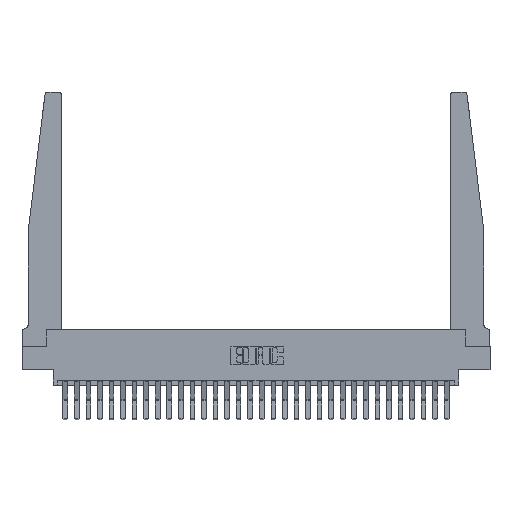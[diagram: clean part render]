
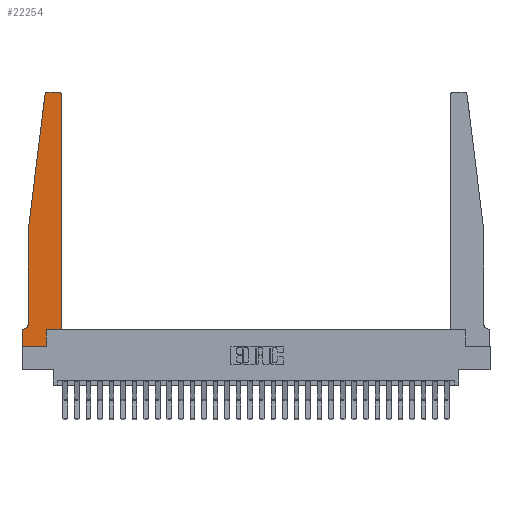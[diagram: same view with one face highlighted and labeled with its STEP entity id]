
A CAD part, top view. The second image highlights one B-rep face of the part: STEP entity #22254.
In plain terms, the highlighted planar face has unit normal (0, 0, 1).
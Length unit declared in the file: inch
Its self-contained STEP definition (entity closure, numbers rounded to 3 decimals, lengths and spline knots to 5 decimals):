
#412 = DIRECTION ( 'NONE',  ( -1., 0., 0. ) ) ;
#1048 = CARTESIAN_POINT ( 'NONE',  ( 0.24675, 2.72367, 0.37 ) ) ;
#1171 = VECTOR ( 'NONE', #17797, 39.37008 ) ;
#1182 = ORIENTED_EDGE ( 'NONE', *, *, #18888, .T. ) ;
#1432 = CARTESIAN_POINT ( 'NONE',  ( 0.015, 0.1875, 0.37 ) ) ;
#1631 = ORIENTED_EDGE ( 'NONE', *, *, #15949, .T. ) ;
#1781 = AXIS2_PLACEMENT_3D ( 'NONE', #4425, #19677, #6575 ) ;
#2222 = PLANE ( 'NONE',  #1781 ) ;
#2535 = EDGE_CURVE ( 'NONE', #12598, #18628, #19215, .T. ) ;
#2574 = CARTESIAN_POINT ( 'NONE',  ( 0.425, 0.18, 0.37 ) ) ;
#3035 = DIRECTION ( 'NONE',  ( 0., 1., 0. ) ) ;
#3255 = VECTOR ( 'NONE', #15378, 39.37008 ) ;
#3931 = LINE ( 'NONE', #6574, #3255 ) ;
#4401 = VERTEX_POINT ( 'NONE', #5819 ) ;
#4425 = CARTESIAN_POINT ( 'NONE',  ( 0., 0.1875, 0.37 ) ) ;
#4804 = ORIENTED_EDGE ( 'NONE', *, *, #23643, .T. ) ;
#4935 = DIRECTION ( 'NONE',  ( 0., -1., 0. ) ) ;
#5178 = VECTOR ( 'NONE', #412, 39.37008 ) ;
#5334 = EDGE_CURVE ( 'NONE', #24561, #4401, #14353, .T. ) ;
#5622 = VERTEX_POINT ( 'NONE', #8802 ) ;
#5819 = CARTESIAN_POINT ( 'NONE',  ( 0.2605, 0.18, 0.37 ) ) ;
#6364 = EDGE_CURVE ( 'NONE', #5622, #7154, #12921, .T. ) ;
#6537 = FACE_OUTER_BOUND ( 'NONE', #28158, .T. ) ;
#6574 = CARTESIAN_POINT ( 'NONE',  ( 0.425, 0.18, 0.37 ) ) ;
#6575 = DIRECTION ( 'NONE',  ( 1., 0., 0. ) ) ;
#7086 = VECTOR ( 'NONE', #15742, 39.37008 ) ;
#7107 = CARTESIAN_POINT ( 'NONE',  ( 0.065, 1.25, 0.37 ) ) ;
#7154 = VERTEX_POINT ( 'NONE', #14189 ) ;
#7252 = CARTESIAN_POINT ( 'NONE',  ( 0.27653, 2.72, 0.37 ) ) ;
#7604 = VECTOR ( 'NONE', #4935, 39.37008 ) ;
#7859 = VECTOR ( 'NONE', #20380, 39.37008 ) ;
#7932 = DIRECTION ( 'NONE',  ( 0., 0., 1. ) ) ;
#8140 = ORIENTED_EDGE ( 'NONE', *, *, #16563, .T. ) ;
#8578 = VERTEX_POINT ( 'NONE', #1432 ) ;
#8802 = CARTESIAN_POINT ( 'NONE',  ( 0.425, 0.18, 0.37 ) ) ;
#9468 = DIRECTION ( 'NONE',  ( 1., 0., 0. ) ) ;
#9746 = CARTESIAN_POINT ( 'NONE',  ( 0.27653, 2.75, 0.37 ) ) ;
#9962 = LINE ( 'NONE', #21421, #20895 ) ;
#11120 = VECTOR ( 'NONE', #24467, 39.37008 ) ;
#11177 = CARTESIAN_POINT ( 'NONE',  ( 0.2605, 0., 0.37 ) ) ;
#11211 = EDGE_CURVE ( 'NONE', #4401, #5622, #3931, .T. ) ;
#11374 = EDGE_CURVE ( 'NONE', #24671, #11467, #23013, .T. ) ;
#11386 = ORIENTED_EDGE ( 'NONE', *, *, #11374, .T. ) ;
#11467 = VERTEX_POINT ( 'NONE', #1048 ) ;
#11608 = CIRCLE ( 'NONE', #27369, 0.05 ) ;
#11744 = VERTEX_POINT ( 'NONE', #21482 ) ;
#11816 = LINE ( 'NONE', #7107, #11120 ) ;
#11883 = CARTESIAN_POINT ( 'NONE',  ( 0.015, 0.2375, 0.37 ) ) ;
#11953 = ORIENTED_EDGE ( 'NONE', *, *, #2535, .T. ) ;
#12598 = VERTEX_POINT ( 'NONE', #24790 ) ;
#12805 = LINE ( 'NONE', #15581, #1171 ) ;
#12921 = LINE ( 'NONE', #2574, #7086 ) ;
#12975 = ORIENTED_EDGE ( 'NONE', *, *, #5334, .T. ) ;
#14073 = DIRECTION ( 'NONE',  ( -1., 0., 0. ) ) ;
#14189 = CARTESIAN_POINT ( 'NONE',  ( 0.425, 2.72, 0.37 ) ) ;
#14353 = LINE ( 'NONE', #16079, #25237 ) ;
#14684 = CARTESIAN_POINT ( 'NONE',  ( 0.395, 2.72, 0.37 ) ) ;
#15039 = LINE ( 'NONE', #15979, #7859 ) ;
#15083 = EDGE_CURVE ( 'NONE', #7154, #11744, #25820, .T. ) ;
#15378 = DIRECTION ( 'NONE',  ( 1., 0., 0. ) ) ;
#15409 = VERTEX_POINT ( 'NONE', #19743 ) ;
#15581 = CARTESIAN_POINT ( 'NONE',  ( 0.065, 0.1875, 0.37 ) ) ;
#15742 = DIRECTION ( 'NONE',  ( 0., 1., 0. ) ) ;
#15809 = CARTESIAN_POINT ( 'NONE',  ( 0.065, 1.25, 0.37 ) ) ;
#15949 = EDGE_CURVE ( 'NONE', #11467, #12598, #11816, .T. ) ;
#15979 = CARTESIAN_POINT ( 'NONE',  ( 0., 0., 0.37 ) ) ;
#16072 = AXIS2_PLACEMENT_3D ( 'NONE', #7252, #22529, #9468 ) ;
#16079 = CARTESIAN_POINT ( 'NONE',  ( 0.2605, 0.18, 0.37 ) ) ;
#16176 = ORIENTED_EDGE ( 'NONE', *, *, #11211, .T. ) ;
#16342 = ORIENTED_EDGE ( 'NONE', *, *, #15083, .T. ) ;
#16563 = EDGE_CURVE ( 'NONE', #8578, #17237, #12805, .T. ) ;
#16910 = ORIENTED_EDGE ( 'NONE', *, *, #6364, .T. ) ;
#17237 = VERTEX_POINT ( 'NONE', #24034 ) ;
#17797 = DIRECTION ( 'NONE',  ( -1., 0., 0. ) ) ;
#18628 = VERTEX_POINT ( 'NONE', #21384 ) ;
#18888 = EDGE_CURVE ( 'NONE', #11744, #24671, #22590, .T. ) ;
#19215 = LINE ( 'NONE', #15809, #7604 ) ;
#19677 = DIRECTION ( 'NONE',  ( 0., 0., 1. ) ) ;
#19743 = CARTESIAN_POINT ( 'NONE',  ( 0., 0., 0.37 ) ) ;
#20380 = DIRECTION ( 'NONE',  ( 1., 0., 0. ) ) ;
#20895 = VECTOR ( 'NONE', #23592, 39.37008 ) ;
#21384 = CARTESIAN_POINT ( 'NONE',  ( 0.065, 0.2375, 0.37 ) ) ;
#21421 = CARTESIAN_POINT ( 'NONE',  ( 0., 0., 0.37 ) ) ;
#21482 = CARTESIAN_POINT ( 'NONE',  ( 0.395, 2.75, 0.37 ) ) ;
#22254 = ADVANCED_FACE ( 'NONE', ( #6537 ), #2222, .T. ) ;
#22338 = AXIS2_PLACEMENT_3D ( 'NONE', #14684, #7932, #23190 ) ;
#22529 = DIRECTION ( 'NONE',  ( 0., 0., 1. ) ) ;
#22590 = LINE ( 'NONE', #26562, #5178 ) ;
#23013 = CIRCLE ( 'NONE', #16072, 0.03 ) ;
#23190 = DIRECTION ( 'NONE',  ( 1., 0., 0. ) ) ;
#23419 = ORIENTED_EDGE ( 'NONE', *, *, #24174, .T. ) ;
#23592 = DIRECTION ( 'NONE',  ( 0., -1., 0. ) ) ;
#23643 = EDGE_CURVE ( 'NONE', #15409, #24561, #15039, .T. ) ;
#23913 = ORIENTED_EDGE ( 'NONE', *, *, #28004, .T. ) ;
#24034 = CARTESIAN_POINT ( 'NONE',  ( 0., 0.1875, 0.37 ) ) ;
#24174 = EDGE_CURVE ( 'NONE', #18628, #8578, #11608, .T. ) ;
#24467 = DIRECTION ( 'NONE',  ( -0.122, -0.992, 0. ) ) ;
#24561 = VERTEX_POINT ( 'NONE', #11177 ) ;
#24671 = VERTEX_POINT ( 'NONE', #9746 ) ;
#24790 = CARTESIAN_POINT ( 'NONE',  ( 0.065, 1.25, 0.37 ) ) ;
#25237 = VECTOR ( 'NONE', #3035, 39.37008 ) ;
#25820 = CIRCLE ( 'NONE', #22338, 0.03 ) ;
#26562 = CARTESIAN_POINT ( 'NONE',  ( 0.25, 2.75, 0.37 ) ) ;
#27093 = DIRECTION ( 'NONE',  ( 0., 0., -1. ) ) ;
#27369 = AXIS2_PLACEMENT_3D ( 'NONE', #11883, #27093, #14073 ) ;
#28004 = EDGE_CURVE ( 'NONE', #17237, #15409, #9962, .T. ) ;
#28158 = EDGE_LOOP ( 'NONE', ( #1182, #11386, #1631, #11953, #23419, #8140, #23913, #4804, #12975, #16176, #16910, #16342 ) ) ;
